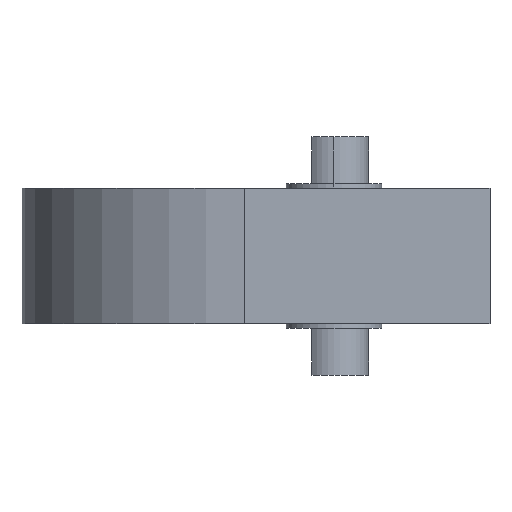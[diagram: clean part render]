
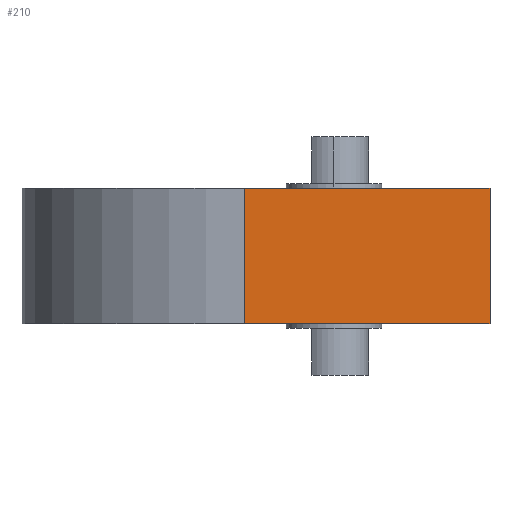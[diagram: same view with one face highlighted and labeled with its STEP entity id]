
A CAD part, left-side view. The second image highlights one B-rep face of the part: STEP entity #210.
In plain terms, the highlighted planar face has unit normal (-1, 0, 0).
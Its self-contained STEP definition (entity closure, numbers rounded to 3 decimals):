
#12 = CARTESIAN_POINT ( 'NONE',  ( 0., 0., 0. ) ) ;
#31 = CARTESIAN_POINT ( 'NONE',  ( 0., 0., 0. ) ) ;
#44 = CARTESIAN_POINT ( 'NONE',  ( 0., 27.94, -15.494 ) ) ;
#69 = ORIENTED_EDGE ( 'NONE', *, *, #605, .F. ) ;
#102 = ORIENTED_EDGE ( 'NONE', *, *, #808, .T. ) ;
#123 = FACE_OUTER_BOUND ( 'NONE', #574, .T. ) ;
#132 = DIRECTION ( 'NONE',  ( 0., 1., 0. ) ) ;
#210 = ADVANCED_FACE ( 'NONE', ( #123 ), #300, .T. ) ;
#270 = VERTEX_POINT ( 'NONE', #44 ) ;
#300 = PLANE ( 'NONE',  #647 ) ;
#452 = VERTEX_POINT ( 'NONE', #1500 ) ;
#515 = CARTESIAN_POINT ( 'NONE',  ( 0., 27.94, 0. ) ) ;
#574 = EDGE_LOOP ( 'NONE', ( #69, #102, #1457, #731 ) ) ;
#605 = EDGE_CURVE ( 'NONE', #1281, #452, #1084, .T. ) ;
#640 = DIRECTION ( 'NONE',  ( 0., 0., -1. ) ) ;
#647 = AXIS2_PLACEMENT_3D ( 'NONE', #31, #1629, #1613 ) ;
#695 = CARTESIAN_POINT ( 'NONE',  ( 0., 0., -15.494 ) ) ;
#699 = VECTOR ( 'NONE', #640, 1000. ) ;
#731 = ORIENTED_EDGE ( 'NONE', *, *, #753, .F. ) ;
#753 = EDGE_CURVE ( 'NONE', #452, #886, #1001, .T. ) ;
#808 = EDGE_CURVE ( 'NONE', #1281, #270, #879, .T. ) ;
#814 = DIRECTION ( 'NONE',  ( 0., 0., -1. ) ) ;
#827 = CARTESIAN_POINT ( 'NONE',  ( 0., 0., -15.494 ) ) ;
#879 = LINE ( 'NONE', #515, #699 ) ;
#886 = VERTEX_POINT ( 'NONE', #695 ) ;
#897 = VECTOR ( 'NONE', #814, 1000. ) ;
#1001 = LINE ( 'NONE', #827, #897 ) ;
#1028 = VECTOR ( 'NONE', #1553, 1000. ) ;
#1029 = EDGE_CURVE ( 'NONE', #886, #270, #1408, .T. ) ;
#1070 = CARTESIAN_POINT ( 'NONE',  ( 0., 27.94, 0. ) ) ;
#1084 = LINE ( 'NONE', #12, #1028 ) ;
#1281 = VERTEX_POINT ( 'NONE', #1070 ) ;
#1336 = VECTOR ( 'NONE', #132, 1000. ) ;
#1408 = LINE ( 'NONE', #1643, #1336 ) ;
#1457 = ORIENTED_EDGE ( 'NONE', *, *, #1029, .F. ) ;
#1500 = CARTESIAN_POINT ( 'NONE',  ( 0., 0., 0. ) ) ;
#1553 = DIRECTION ( 'NONE',  ( 0., -1., 0. ) ) ;
#1613 = DIRECTION ( 'NONE',  ( 0., 0., 1. ) ) ;
#1629 = DIRECTION ( 'NONE',  ( -1., 0., 0. ) ) ;
#1643 = CARTESIAN_POINT ( 'NONE',  ( 0., 25.4, -15.494 ) ) ;
